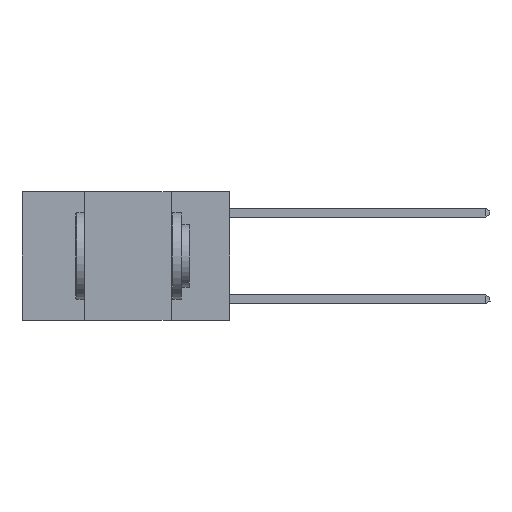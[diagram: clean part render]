
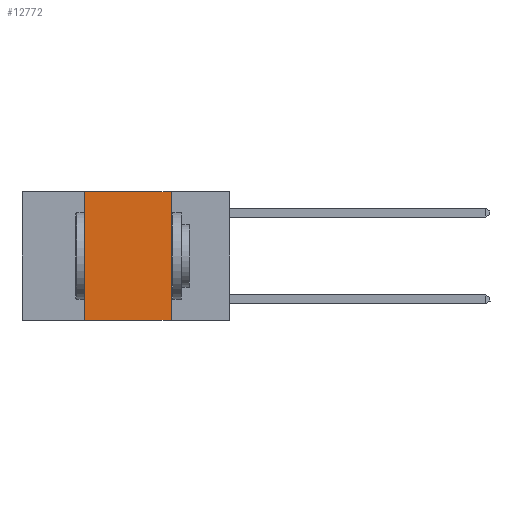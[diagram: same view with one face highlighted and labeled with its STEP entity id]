
A CAD part, left-side view. The second image highlights one B-rep face of the part: STEP entity #12772.
In plain terms, the highlighted planar face has unit normal (-1, 0, 0).
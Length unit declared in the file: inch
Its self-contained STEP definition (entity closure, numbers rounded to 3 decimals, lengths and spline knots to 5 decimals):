
#423 = CARTESIAN_POINT ( 'NONE',  ( 0., 0.42, -0.37 ) ) ;
#628 = FACE_OUTER_BOUND ( 'NONE', #1531, .T. ) ;
#1425 = CARTESIAN_POINT ( 'NONE',  ( 0., 0.17, -0.37 ) ) ;
#1531 = EDGE_LOOP ( 'NONE', ( #10548, #9771, #6636, #13291 ) ) ;
#1847 = DIRECTION ( 'NONE',  ( 0., 0., -1. ) ) ;
#2445 = CARTESIAN_POINT ( 'NONE',  ( 0., 0.42, 0. ) ) ;
#2808 = CARTESIAN_POINT ( 'NONE',  ( 0., 0.42, 0. ) ) ;
#4266 = CARTESIAN_POINT ( 'NONE',  ( 0., 0.6, -0.37 ) ) ;
#5875 = DIRECTION ( 'NONE',  ( 0., -1., 0. ) ) ;
#6161 = VECTOR ( 'NONE', #11458, 39.37008 ) ;
#6440 = PLANE ( 'NONE',  #7704 ) ;
#6636 = ORIENTED_EDGE ( 'NONE', *, *, #11493, .F. ) ;
#7660 = VECTOR ( 'NONE', #1847, 39.37008 ) ;
#7704 = AXIS2_PLACEMENT_3D ( 'NONE', #18056, #9388, #15093 ) ;
#8713 = LINE ( 'NONE', #4266, #11477 ) ;
#8718 = CARTESIAN_POINT ( 'NONE',  ( 0., 0.17, 0. ) ) ;
#9066 = CARTESIAN_POINT ( 'NONE',  ( 0., 0.17, 0. ) ) ;
#9388 = DIRECTION ( 'NONE',  ( 1., 0., 0. ) ) ;
#9503 = VECTOR ( 'NONE', #5875, 39.37008 ) ;
#9771 = ORIENTED_EDGE ( 'NONE', *, *, #11252, .F. ) ;
#9903 = EDGE_CURVE ( 'NONE', #12465, #12000, #13359, .T. ) ;
#10548 = ORIENTED_EDGE ( 'NONE', *, *, #9903, .F. ) ;
#11252 = EDGE_CURVE ( 'NONE', #14204, #12465, #14720, .T. ) ;
#11458 = DIRECTION ( 'NONE',  ( 0., 0., 1. ) ) ;
#11477 = VECTOR ( 'NONE', #13201, 39.37008 ) ;
#11493 = EDGE_CURVE ( 'NONE', #14441, #14204, #14312, .T. ) ;
#12000 = VERTEX_POINT ( 'NONE', #1425 ) ;
#12465 = VERTEX_POINT ( 'NONE', #8718 ) ;
#12772 = ADVANCED_FACE ( 'NONE', ( #628 ), #6440, .F. ) ;
#13201 = DIRECTION ( 'NONE',  ( 0., -1., 0. ) ) ;
#13291 = ORIENTED_EDGE ( 'NONE', *, *, #16741, .T. ) ;
#13359 = LINE ( 'NONE', #9066, #7660 ) ;
#14204 = VERTEX_POINT ( 'NONE', #2808 ) ;
#14312 = LINE ( 'NONE', #2445, #6161 ) ;
#14441 = VERTEX_POINT ( 'NONE', #423 ) ;
#14720 = LINE ( 'NONE', #14808, #9503 ) ;
#14808 = CARTESIAN_POINT ( 'NONE',  ( 0., 0.6, 0. ) ) ;
#15093 = DIRECTION ( 'NONE',  ( 0., 0., -1. ) ) ;
#16741 = EDGE_CURVE ( 'NONE', #14441, #12000, #8713, .T. ) ;
#18056 = CARTESIAN_POINT ( 'NONE',  ( 0., 0.6, 0. ) ) ;
